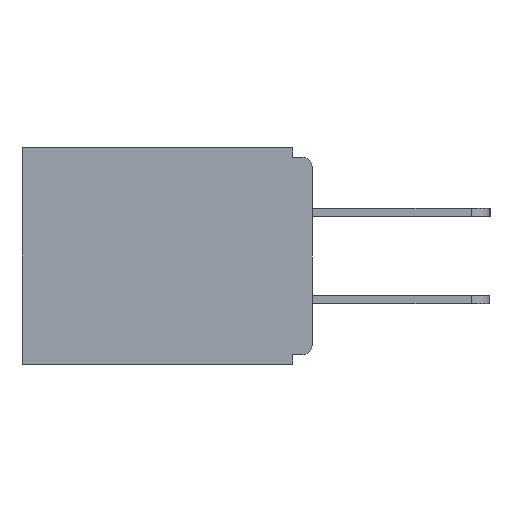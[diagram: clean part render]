
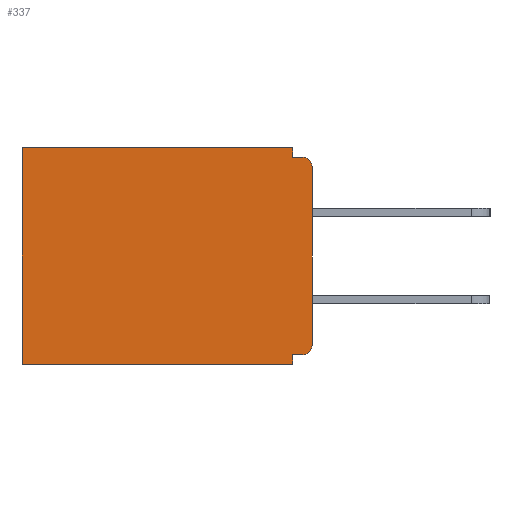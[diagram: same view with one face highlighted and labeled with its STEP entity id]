
A CAD part, left-side view. The second image highlights one B-rep face of the part: STEP entity #337.
In plain terms, the highlighted planar face has unit normal (-1, 0, 0).
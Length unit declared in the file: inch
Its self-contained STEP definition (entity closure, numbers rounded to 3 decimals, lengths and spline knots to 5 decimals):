
#212 = CARTESIAN_POINT ( 'NONE',  ( 0.298, 0., -0.313 ) ) ;
#337 = ADVANCED_FACE ( 'NONE', ( #11924 ), #4786, .F. ) ;
#347 = VECTOR ( 'NONE', #10551, 39.37008 ) ;
#356 = CARTESIAN_POINT ( 'NONE',  ( 0.298, 0.015, -0.03 ) ) ;
#495 = DIRECTION ( 'NONE',  ( 0., -1., 0. ) ) ;
#1161 = EDGE_CURVE ( 'NONE', #10822, #18005, #7963, .T. ) ;
#1359 = CARTESIAN_POINT ( 'NONE',  ( 0.298, 0., -0.343 ) ) ;
#1863 = EDGE_CURVE ( 'NONE', #8320, #4619, #2667, .T. ) ;
#1976 = CARTESIAN_POINT ( 'NONE',  ( 0.298, 0.015, -0.328 ) ) ;
#2027 = AXIS2_PLACEMENT_3D ( 'NONE', #10720, #16571, #3268 ) ;
#2031 = ORIENTED_EDGE ( 'NONE', *, *, #1161, .T. ) ;
#2467 = CARTESIAN_POINT ( 'NONE',  ( 0.298, 0., 0. ) ) ;
#2533 = CARTESIAN_POINT ( 'NONE',  ( 0.298, 0.015, -0.313 ) ) ;
#2667 = LINE ( 'NONE', #13453, #13530 ) ;
#3019 = DIRECTION ( 'NONE',  ( 0., 1., 0. ) ) ;
#3268 = DIRECTION ( 'NONE',  ( 0., 0., -1. ) ) ;
#3419 = VECTOR ( 'NONE', #3019, 39.37008 ) ;
#3566 = ORIENTED_EDGE ( 'NONE', *, *, #8355, .F. ) ;
#3835 = DIRECTION ( 'NONE',  ( 0., 1., 0. ) ) ;
#3911 = AXIS2_PLACEMENT_3D ( 'NONE', #2533, #14408, #7000 ) ;
#4462 = CARTESIAN_POINT ( 'NONE',  ( 0.298, 0.46, 0. ) ) ;
#4619 = VERTEX_POINT ( 'NONE', #4770 ) ;
#4770 = CARTESIAN_POINT ( 'NONE',  ( 0.298, 0.031, -0.015 ) ) ;
#4786 = PLANE ( 'NONE',  #2027 ) ;
#4789 = VERTEX_POINT ( 'NONE', #212 ) ;
#4853 = VERTEX_POINT ( 'NONE', #6740 ) ;
#5007 = LINE ( 'NONE', #18389, #12393 ) ;
#5130 = LINE ( 'NONE', #2467, #11126 ) ;
#6469 = ORIENTED_EDGE ( 'NONE', *, *, #17667, .T. ) ;
#6740 = CARTESIAN_POINT ( 'NONE',  ( 0.298, 0.015, -0.015 ) ) ;
#7000 = DIRECTION ( 'NONE',  ( 0., 0., -1. ) ) ;
#7376 = VECTOR ( 'NONE', #3835, 39.37008 ) ;
#7963 = LINE ( 'NONE', #10927, #15667 ) ;
#8314 = EDGE_CURVE ( 'NONE', #14066, #18005, #11464, .T. ) ;
#8320 = VERTEX_POINT ( 'NONE', #12614 ) ;
#8355 = EDGE_CURVE ( 'NONE', #15248, #4789, #10559, .T. ) ;
#9074 = CARTESIAN_POINT ( 'NONE',  ( 0.298, 0., 0. ) ) ;
#9086 = VECTOR ( 'NONE', #495, 39.37008 ) ;
#9302 = CIRCLE ( 'NONE', #3911, 0.015 ) ;
#9908 = ORIENTED_EDGE ( 'NONE', *, *, #11347, .F. ) ;
#10063 = ORIENTED_EDGE ( 'NONE', *, *, #13828, .T. ) ;
#10332 = ORIENTED_EDGE ( 'NONE', *, *, #8314, .F. ) ;
#10454 = LINE ( 'NONE', #12331, #9086 ) ;
#10513 = AXIS2_PLACEMENT_3D ( 'NONE', #356, #10657, #12145 ) ;
#10551 = DIRECTION ( 'NONE',  ( 0., 0., -1. ) ) ;
#10559 = LINE ( 'NONE', #9074, #347 ) ;
#10657 = DIRECTION ( 'NONE',  ( -1., 0., 0. ) ) ;
#10720 = CARTESIAN_POINT ( 'NONE',  ( 0.298, 0., 0. ) ) ;
#10822 = VERTEX_POINT ( 'NONE', #4462 ) ;
#10927 = CARTESIAN_POINT ( 'NONE',  ( 0.298, 0.46, 0. ) ) ;
#11017 = VERTEX_POINT ( 'NONE', #15784 ) ;
#11126 = VECTOR ( 'NONE', #16624, 39.37008 ) ;
#11218 = DIRECTION ( 'NONE',  ( 0., 0., -1. ) ) ;
#11347 = EDGE_CURVE ( 'NONE', #11017, #14066, #5007, .T. ) ;
#11374 = ORIENTED_EDGE ( 'NONE', *, *, #17984, .F. ) ;
#11464 = LINE ( 'NONE', #1359, #3419 ) ;
#11486 = ORIENTED_EDGE ( 'NONE', *, *, #17194, .F. ) ;
#11924 = FACE_OUTER_BOUND ( 'NONE', #16657, .T. ) ;
#12080 = EDGE_CURVE ( 'NONE', #15248, #4853, #17796, .T. ) ;
#12145 = DIRECTION ( 'NONE',  ( 0., 0., -1. ) ) ;
#12173 = CARTESIAN_POINT ( 'NONE',  ( 0.298, 0.031, -0.343 ) ) ;
#12243 = ORIENTED_EDGE ( 'NONE', *, *, #1863, .F. ) ;
#12331 = CARTESIAN_POINT ( 'NONE',  ( 0.298, 0., -0.015 ) ) ;
#12393 = VECTOR ( 'NONE', #11218, 39.37008 ) ;
#12614 = CARTESIAN_POINT ( 'NONE',  ( 0.298, 0.031, 0. ) ) ;
#13453 = CARTESIAN_POINT ( 'NONE',  ( 0.298, 0.031, -0.343 ) ) ;
#13530 = VECTOR ( 'NONE', #16505, 39.37008 ) ;
#13828 = EDGE_CURVE ( 'NONE', #8320, #10822, #5130, .T. ) ;
#14066 = VERTEX_POINT ( 'NONE', #12173 ) ;
#14142 = CARTESIAN_POINT ( 'NONE',  ( 0.298, 0.46, -0.343 ) ) ;
#14172 = VERTEX_POINT ( 'NONE', #1976 ) ;
#14404 = CARTESIAN_POINT ( 'NONE',  ( 0.298, 0., -0.328 ) ) ;
#14408 = DIRECTION ( 'NONE',  ( -1., 0., 0. ) ) ;
#15248 = VERTEX_POINT ( 'NONE', #16371 ) ;
#15667 = VECTOR ( 'NONE', #16367, 39.37008 ) ;
#15784 = CARTESIAN_POINT ( 'NONE',  ( 0.298, 0.031, -0.328 ) ) ;
#16367 = DIRECTION ( 'NONE',  ( 0., 0., -1. ) ) ;
#16371 = CARTESIAN_POINT ( 'NONE',  ( 0.298, 0., -0.03 ) ) ;
#16505 = DIRECTION ( 'NONE',  ( 0., 0., -1. ) ) ;
#16571 = DIRECTION ( 'NONE',  ( 1., 0., 0. ) ) ;
#16624 = DIRECTION ( 'NONE',  ( 0., 1., 0. ) ) ;
#16657 = EDGE_LOOP ( 'NONE', ( #16732, #11486, #12243, #10063, #2031, #10332, #9908, #11374, #6469, #3566 ) ) ;
#16732 = ORIENTED_EDGE ( 'NONE', *, *, #12080, .T. ) ;
#17194 = EDGE_CURVE ( 'NONE', #4619, #4853, #10454, .T. ) ;
#17667 = EDGE_CURVE ( 'NONE', #14172, #4789, #9302, .T. ) ;
#17796 = CIRCLE ( 'NONE', #10513, 0.015 ) ;
#17984 = EDGE_CURVE ( 'NONE', #14172, #11017, #18623, .T. ) ;
#18005 = VERTEX_POINT ( 'NONE', #14142 ) ;
#18389 = CARTESIAN_POINT ( 'NONE',  ( 0.298, 0.031, -0.343 ) ) ;
#18623 = LINE ( 'NONE', #14404, #7376 ) ;
